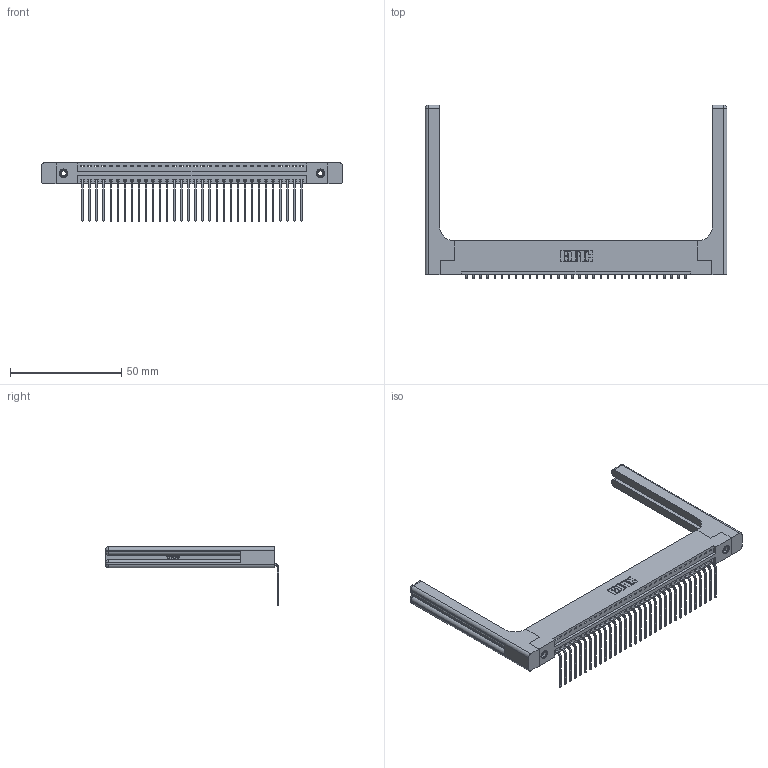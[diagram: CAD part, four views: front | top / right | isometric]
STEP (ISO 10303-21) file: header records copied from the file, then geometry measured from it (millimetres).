
FILE_DESCRIPTION (( 'STEP AP203' ), '1' );
FILE_NAME ('396-032-559-158.STEP', '2019-10-31T22:00:03', ( '' ), ( '' ), 'SwSTEP 2.0', 'SolidWorks 2016', '' );
FILE_SCHEMA (( 'CONFIG_CONTROL_DESIGN' ));
Length unit declared in the file: inch
Products named in the file (5): 345-292-001_558 559 Tail - 1; 345-250-001_345-250-001-102; 346-220-058_345-220-058; 396-032-559-158; 346 Part_Flush Mounting Lugs - 0.156 Dia-TH
Assembly tree (37 placements, depth 2):
  396-032-559-158
    346 Part_Flush Mounting Lugs - 0.156 Dia-TH
    345-292-001_558 559 Tail - 1  x32
    345-250-001_345-250-001-102  x2
    346-220-058_345-220-058  x2
Bounding box: 135.66 x 78.04 x 26.16 mm (x, y, z)
Volume: 20541.9 mm3; surface area: 21975.4 mm2
Topology: 37 solids, 37 shells, 2298 faces, 6819 edges, 4482 vertices
Faces by surface type: plane 1568, cylinder 670, bspline 36, cone 12, sphere 8, torus 4
Entity records: 26472 total; most frequent: CARTESIAN_POINT 5521, ORIENTED_EDGE 4284, DIRECTION 3814, EDGE_CURVE 2142, VECTOR 1790, LINE 1790, VERTEX_POINT 1418, AXIS2_PLACEMENT_3D 1012
